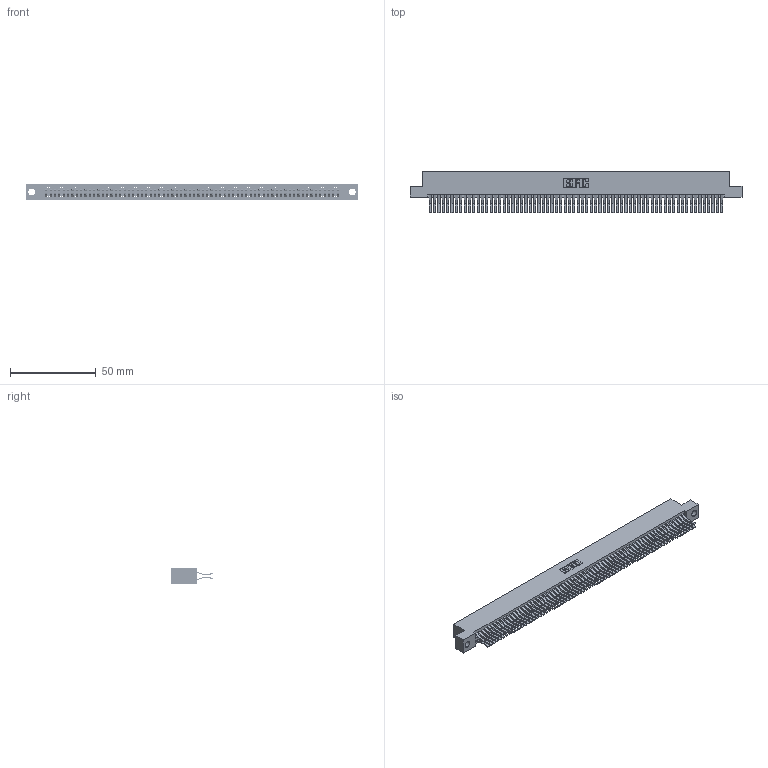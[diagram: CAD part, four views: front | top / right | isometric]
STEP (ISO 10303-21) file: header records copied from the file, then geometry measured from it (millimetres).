
FILE_DESCRIPTION (( 'STEP AP203' ), '1' );
FILE_NAME ('345-136-560-204.STEP', '2018-10-20T16:20:44', ( '' ), ( '' ), 'SwSTEP 2.0', 'SolidWorks 2016', '' );
FILE_SCHEMA (( 'CONFIG_CONTROL_DESIGN' ));
Length unit declared in the file: inch
Products named in the file (3): 345-136-560-204; 345-292-001_560 Tail; 345 Part_Flush Mounting Lugs - 0.156 Dia-TH
Assembly tree (137 placements, depth 2):
  345-136-560-204
    345 Part_Flush Mounting Lugs - 0.156 Dia-TH
    345-292-001_560 Tail  x136
Bounding box: 193.93 x 24.45 x 9.4 mm (x, y, z)
Volume: 19883.4 mm3; surface area: 32002.4 mm2
Topology: 137 solids, 137 shells, 7198 faces, 21421 edges, 14098 vertices
Faces by surface type: plane 4568, cylinder 2630
Entity records: 49945 total; most frequent: CARTESIAN_POINT 8348, ORIENTED_EDGE 8282, DIRECTION 7333, EDGE_CURVE 4141, LINE 3733, VECTOR 3733, VERTEX_POINT 2758, AXIS2_PLACEMENT_3D 1800
